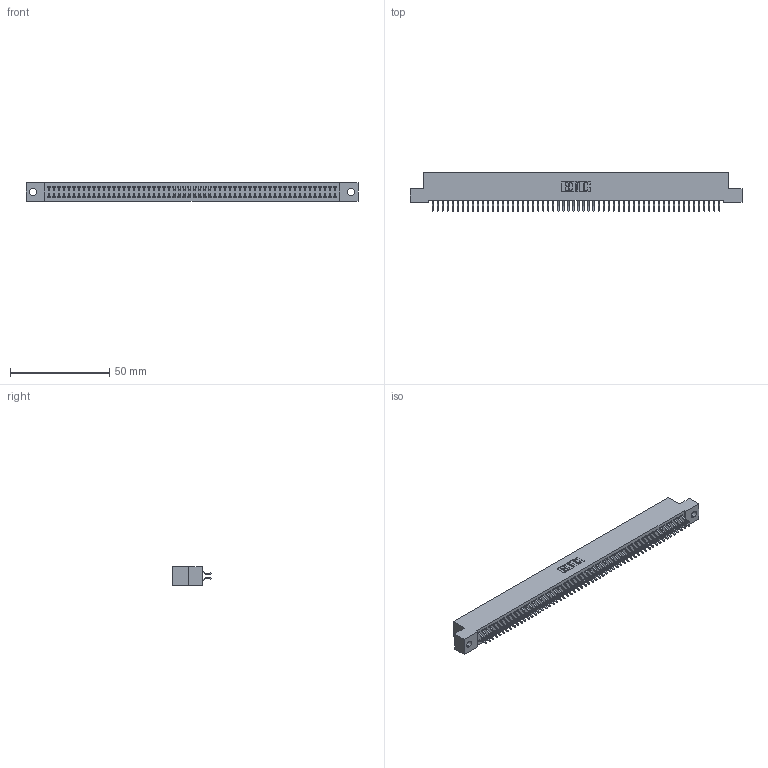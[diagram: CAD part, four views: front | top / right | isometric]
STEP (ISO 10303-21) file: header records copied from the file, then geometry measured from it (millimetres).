
FILE_DESCRIPTION (( 'STEP AP203' ), '1' );
FILE_NAME ('392-116-556-202.STEP', '2018-08-19T00:22:19', ( '' ), ( '' ), 'SwSTEP 2.0', 'SolidWorks 2016', '' );
FILE_SCHEMA (( 'CONFIG_CONTROL_DESIGN' ));
Length unit declared in the file: inch
Products named in the file (3): 342 Part_.128 Slot; 345-292-001_556 Tail; 392-116-556-202
Assembly tree (117 placements, depth 2):
  392-116-556-202
    342 Part_.128 Slot
    345-292-001_556 Tail  x116
Bounding box: 167.64 x 19.58 x 9.4 mm (x, y, z)
Volume: 15083.1 mm3; surface area: 24592.7 mm2
Topology: 117 solids, 117 shells, 6842 faces, 20379 edges, 13430 vertices
Faces by surface type: plane 4710, cylinder 2132
Entity records: 35467 total; most frequent: CARTESIAN_POINT 5874, ORIENTED_EDGE 5798, DIRECTION 4979, EDGE_CURVE 2899, LINE 2763, VECTOR 2763, VERTEX_POINT 1930, AXIS2_PLACEMENT_3D 1108
